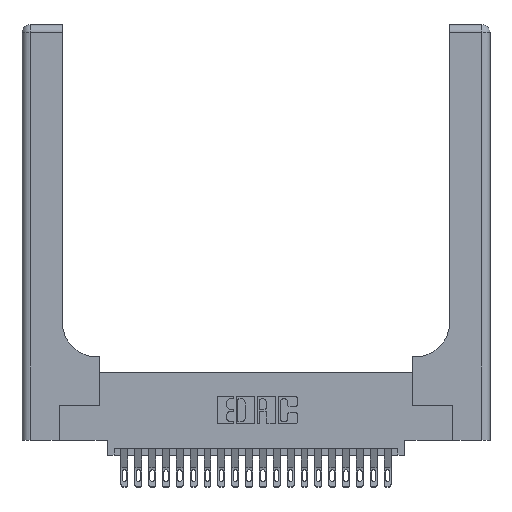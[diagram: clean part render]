
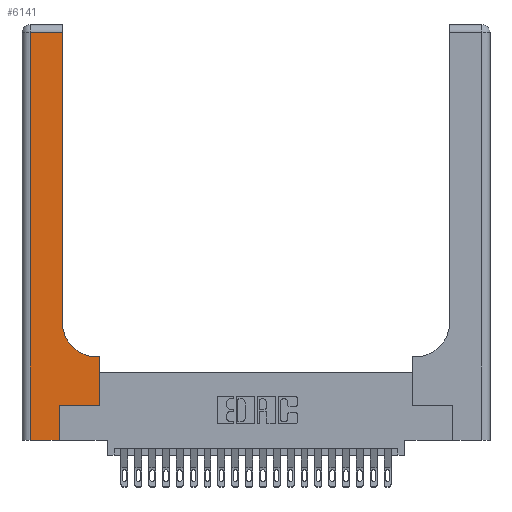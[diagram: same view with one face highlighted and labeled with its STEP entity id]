
A CAD part, top view. The second image highlights one B-rep face of the part: STEP entity #6141.
In plain terms, the highlighted planar face has unit normal (0, 0, 1).
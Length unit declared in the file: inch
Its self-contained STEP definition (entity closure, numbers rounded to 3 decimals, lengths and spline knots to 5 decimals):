
#428 = EDGE_CURVE ( 'NONE', #671, #23314, #16577, .T. ) ;
#671 = VERTEX_POINT ( 'NONE', #19770 ) ;
#1369 = EDGE_LOOP ( 'NONE', ( #7038, #1461, #6541, #12454, #17974, #19795, #9892, #7953, #4254 ) ) ;
#1461 = ORIENTED_EDGE ( 'NONE', *, *, #7793, .T. ) ;
#1702 = CARTESIAN_POINT ( 'NONE',  ( 0., 0., 0.37 ) ) ;
#2198 = LINE ( 'NONE', #11571, #7784 ) ;
#2741 = CARTESIAN_POINT ( 'NONE',  ( 0.5585, 0.25, 0.37 ) ) ;
#3074 = PLANE ( 'NONE',  #8055 ) ;
#4198 = VERTEX_POINT ( 'NONE', #10102 ) ;
#4254 = ORIENTED_EDGE ( 'NONE', *, *, #4492, .T. ) ;
#4492 = EDGE_CURVE ( 'NONE', #13004, #20760, #12103, .T. ) ;
#4629 = CARTESIAN_POINT ( 'NONE',  ( 0.5585, 0.6, 0.37 ) ) ;
#5203 = EDGE_CURVE ( 'NONE', #15633, #7496, #17324, .T. ) ;
#5218 = CARTESIAN_POINT ( 'NONE',  ( 0., 3., 0.37 ) ) ;
#5407 = DIRECTION ( 'NONE',  ( 0., 0., -1. ) ) ;
#5501 = AXIS2_PLACEMENT_3D ( 'NONE', #16646, #5407, #15990 ) ;
#5789 = LINE ( 'NONE', #8941, #18971 ) ;
#6125 = CARTESIAN_POINT ( 'NONE',  ( 0.5415, 0.6, 0.37 ) ) ;
#6141 = ADVANCED_FACE ( 'NONE', ( #16146 ), #3074, .F. ) ;
#6541 = ORIENTED_EDGE ( 'NONE', *, *, #428, .T. ) ;
#7038 = ORIENTED_EDGE ( 'NONE', *, *, #21221, .T. ) ;
#7152 = DIRECTION ( 'NONE',  ( 0., 1., 0. ) ) ;
#7496 = VERTEX_POINT ( 'NONE', #4629 ) ;
#7531 = DIRECTION ( 'NONE',  ( 1., 0., 0. ) ) ;
#7709 = CARTESIAN_POINT ( 'NONE',  ( 0.2915, 0.6, 0.37 ) ) ;
#7784 = VECTOR ( 'NONE', #11807, 39.37008 ) ;
#7793 = EDGE_CURVE ( 'NONE', #17795, #671, #5789, .T. ) ;
#7953 = ORIENTED_EDGE ( 'NONE', *, *, #19719, .T. ) ;
#8055 = AXIS2_PLACEMENT_3D ( 'NONE', #5218, #10885, #22424 ) ;
#8941 = CARTESIAN_POINT ( 'NONE',  ( 0., 2.94, 0.37 ) ) ;
#9195 = DIRECTION ( 'NONE',  ( -1., 0., 0. ) ) ;
#9892 = ORIENTED_EDGE ( 'NONE', *, *, #5203, .T. ) ;
#10102 = CARTESIAN_POINT ( 'NONE',  ( 0.269, 0.25, 0.37 ) ) ;
#10885 = DIRECTION ( 'NONE',  ( 0., 0., -1. ) ) ;
#10911 = CARTESIAN_POINT ( 'NONE',  ( 0.06, 3., 0.37 ) ) ;
#11501 = LINE ( 'NONE', #7709, #20293 ) ;
#11571 = CARTESIAN_POINT ( 'NONE',  ( 0.269, 0., 0.37 ) ) ;
#11807 = DIRECTION ( 'NONE',  ( 0., 1., 0. ) ) ;
#12103 = CIRCLE ( 'NONE', #5501, 0.25 ) ;
#12153 = EDGE_CURVE ( 'NONE', #4198, #15633, #23984, .T. ) ;
#12454 = ORIENTED_EDGE ( 'NONE', *, *, #18152, .T. ) ;
#12531 = CARTESIAN_POINT ( 'NONE',  ( 0.2915, 0.85, 0.37 ) ) ;
#13004 = VERTEX_POINT ( 'NONE', #6125 ) ;
#14858 = CARTESIAN_POINT ( 'NONE',  ( 0.5585, 0.25, 0.37 ) ) ;
#15544 = DIRECTION ( 'NONE',  ( 0., 1., 0. ) ) ;
#15633 = VERTEX_POINT ( 'NONE', #2741 ) ;
#15972 = VECTOR ( 'NONE', #7531, 39.37008 ) ;
#15990 = DIRECTION ( 'NONE',  ( 1., 0., 0. ) ) ;
#16146 = FACE_OUTER_BOUND ( 'NONE', #1369, .T. ) ;
#16577 = LINE ( 'NONE', #10911, #18027 ) ;
#16646 = CARTESIAN_POINT ( 'NONE',  ( 0.5415, 0.85, 0.37 ) ) ;
#17183 = EDGE_CURVE ( 'NONE', #21281, #4198, #2198, .T. ) ;
#17324 = LINE ( 'NONE', #14858, #22644 ) ;
#17566 = VECTOR ( 'NONE', #15544, 39.37008 ) ;
#17795 = VERTEX_POINT ( 'NONE', #22848 ) ;
#17933 = CARTESIAN_POINT ( 'NONE',  ( 0.269, 0., 0.37 ) ) ;
#17974 = ORIENTED_EDGE ( 'NONE', *, *, #17183, .T. ) ;
#18027 = VECTOR ( 'NONE', #20003, 39.37008 ) ;
#18120 = VECTOR ( 'NONE', #19455, 39.37008 ) ;
#18152 = EDGE_CURVE ( 'NONE', #23314, #21281, #19166, .T. ) ;
#18184 = LINE ( 'NONE', #23332, #17566 ) ;
#18971 = VECTOR ( 'NONE', #9195, 39.37008 ) ;
#19166 = LINE ( 'NONE', #1702, #15972 ) ;
#19295 = CARTESIAN_POINT ( 'NONE',  ( 0.269, 0.25, 0.37 ) ) ;
#19455 = DIRECTION ( 'NONE',  ( 1., 0., 0. ) ) ;
#19719 = EDGE_CURVE ( 'NONE', #7496, #13004, #11501, .T. ) ;
#19770 = CARTESIAN_POINT ( 'NONE',  ( 0.06, 2.94, 0.37 ) ) ;
#19795 = ORIENTED_EDGE ( 'NONE', *, *, #12153, .T. ) ;
#20003 = DIRECTION ( 'NONE',  ( 0., -1., 0. ) ) ;
#20293 = VECTOR ( 'NONE', #21169, 39.37008 ) ;
#20760 = VERTEX_POINT ( 'NONE', #12531 ) ;
#21169 = DIRECTION ( 'NONE',  ( -1., 0., 0. ) ) ;
#21221 = EDGE_CURVE ( 'NONE', #20760, #17795, #18184, .T. ) ;
#21281 = VERTEX_POINT ( 'NONE', #17933 ) ;
#22424 = DIRECTION ( 'NONE',  ( -1., 0., 0. ) ) ;
#22644 = VECTOR ( 'NONE', #7152, 39.37008 ) ;
#22848 = CARTESIAN_POINT ( 'NONE',  ( 0.2915, 2.94, 0.37 ) ) ;
#23314 = VERTEX_POINT ( 'NONE', #23348 ) ;
#23332 = CARTESIAN_POINT ( 'NONE',  ( 0.2915, 3., 0.37 ) ) ;
#23348 = CARTESIAN_POINT ( 'NONE',  ( 0.06, 0., 0.37 ) ) ;
#23984 = LINE ( 'NONE', #19295, #18120 ) ;
